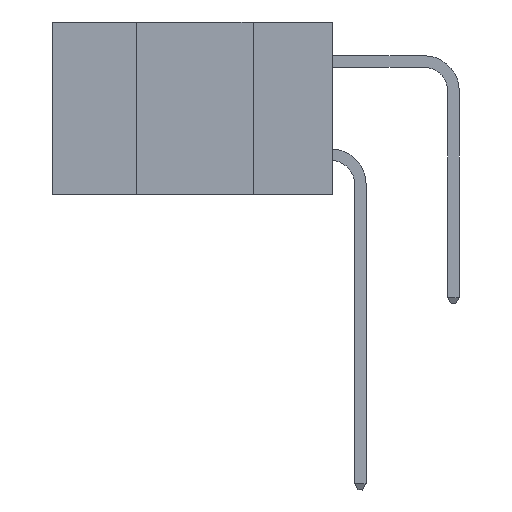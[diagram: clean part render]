
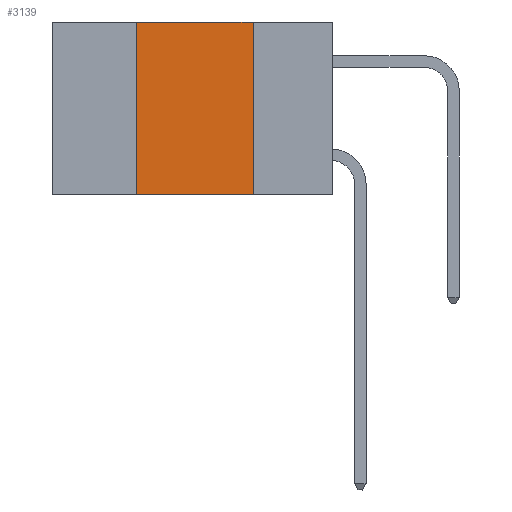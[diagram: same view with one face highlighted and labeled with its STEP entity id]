
A CAD part, left-side view. The second image highlights one B-rep face of the part: STEP entity #3139.
In plain terms, the highlighted planar face has unit normal (-1, 0, 0).
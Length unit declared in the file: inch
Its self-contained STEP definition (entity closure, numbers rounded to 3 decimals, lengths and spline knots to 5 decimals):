
#180 = LINE ( 'NONE', #4790, #13484 ) ;
#328 = ORIENTED_EDGE ( 'NONE', *, *, #21129, .F. ) ;
#1238 = AXIS2_PLACEMENT_3D ( 'NONE', #25754, #13318, #17760 ) ;
#1356 = CARTESIAN_POINT ( 'NONE',  ( 0., 0.42, -0.37 ) ) ;
#1886 = DIRECTION ( 'NONE',  ( 0., 0., -1. ) ) ;
#3139 = ADVANCED_FACE ( 'NONE', ( #8742 ), #10824, .F. ) ;
#3603 = DIRECTION ( 'NONE',  ( 0., 0., 1. ) ) ;
#3699 = EDGE_LOOP ( 'NONE', ( #4689, #5829, #328, #23874 ) ) ;
#3964 = VERTEX_POINT ( 'NONE', #23049 ) ;
#4689 = ORIENTED_EDGE ( 'NONE', *, *, #23010, .F. ) ;
#4790 = CARTESIAN_POINT ( 'NONE',  ( 0., 0.6, -0.37 ) ) ;
#5829 = ORIENTED_EDGE ( 'NONE', *, *, #20868, .F. ) ;
#5903 = CARTESIAN_POINT ( 'NONE',  ( 0., 0.17, -0.37 ) ) ;
#7628 = VERTEX_POINT ( 'NONE', #19988 ) ;
#7662 = LINE ( 'NONE', #1356, #19309 ) ;
#8742 = FACE_OUTER_BOUND ( 'NONE', #3699, .T. ) ;
#9955 = VECTOR ( 'NONE', #10464, 39.37008 ) ;
#10464 = DIRECTION ( 'NONE',  ( 0., -1., 0. ) ) ;
#10824 = PLANE ( 'NONE',  #1238 ) ;
#10873 = LINE ( 'NONE', #19368, #9955 ) ;
#11489 = VERTEX_POINT ( 'NONE', #11668 ) ;
#11668 = CARTESIAN_POINT ( 'NONE',  ( 0., 0.17, 0. ) ) ;
#13030 = DIRECTION ( 'NONE',  ( 0., -1., 0. ) ) ;
#13318 = DIRECTION ( 'NONE',  ( 1., 0., 0. ) ) ;
#13484 = VECTOR ( 'NONE', #13030, 39.37008 ) ;
#16242 = VECTOR ( 'NONE', #1886, 39.37008 ) ;
#16416 = VERTEX_POINT ( 'NONE', #5903 ) ;
#17760 = DIRECTION ( 'NONE',  ( 0., 0., -1. ) ) ;
#18764 = LINE ( 'NONE', #23100, #16242 ) ;
#19309 = VECTOR ( 'NONE', #3603, 39.37008 ) ;
#19368 = CARTESIAN_POINT ( 'NONE',  ( 0., 0.6, 0. ) ) ;
#19988 = CARTESIAN_POINT ( 'NONE',  ( 0., 0.42, 0. ) ) ;
#20025 = EDGE_CURVE ( 'NONE', #3964, #16416, #180, .T. ) ;
#20868 = EDGE_CURVE ( 'NONE', #7628, #11489, #10873, .T. ) ;
#21129 = EDGE_CURVE ( 'NONE', #3964, #7628, #7662, .T. ) ;
#23010 = EDGE_CURVE ( 'NONE', #11489, #16416, #18764, .T. ) ;
#23049 = CARTESIAN_POINT ( 'NONE',  ( 0., 0.42, -0.37 ) ) ;
#23100 = CARTESIAN_POINT ( 'NONE',  ( 0., 0.17, -0.37 ) ) ;
#23874 = ORIENTED_EDGE ( 'NONE', *, *, #20025, .T. ) ;
#25754 = CARTESIAN_POINT ( 'NONE',  ( 0., 0.6, 0. ) ) ;
